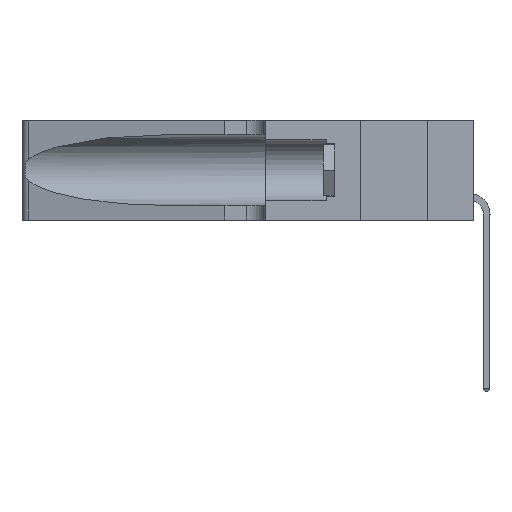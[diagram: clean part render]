
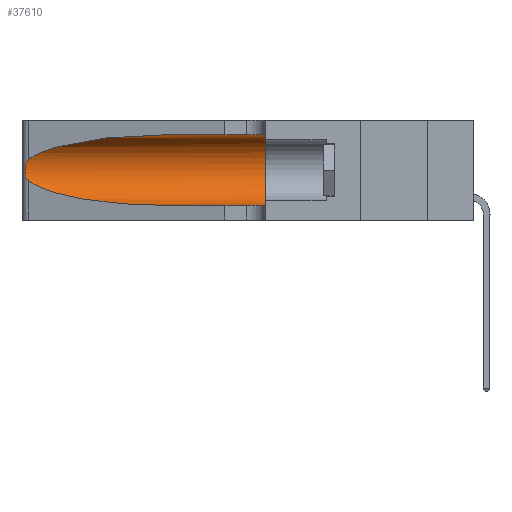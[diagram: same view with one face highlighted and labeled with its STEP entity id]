
A CAD part, left-side view. The second image highlights one B-rep face of the part: STEP entity #37610.
In plain terms, the highlighted cylindrical face has radius 3.308 mm (diameter 6.617 mm), a partial arc.
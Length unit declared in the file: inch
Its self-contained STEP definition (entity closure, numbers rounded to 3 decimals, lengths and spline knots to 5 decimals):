
#437 = CARTESIAN_POINT ( 'NONE',  ( 0.25487, 1.22718, 0.14631 ) ) ;
#970 = VERTEX_POINT ( 'NONE', #36939 ) ;
#1136 = CARTESIAN_POINT ( 'NONE',  ( 0.18966, 0.96281, 0.05475 ) ) ;
#1139 = EDGE_CURVE ( 'NONE', #23087, #42691, #31181, .T. ) ;
#1422 = CARTESIAN_POINT ( 'NONE',  ( 0.2373, 1.15595, 0.08982 ) ) ;
#1552 = ORIENTED_EDGE ( 'NONE', *, *, #41452, .T. ) ;
#1621 = EDGE_CURVE ( 'NONE', #970, #6947, #23301, .T. ) ;
#2358 = CARTESIAN_POINT ( 'NONE',  ( 0.25487, 1.22718, 0.22369 ) ) ;
#2500 = CARTESIAN_POINT ( 'NONE',  ( 0.25639, 1.23186, 0.15144 ) ) ;
#2774 = CARTESIAN_POINT ( 'NONE',  ( 0.1305, 1.61858, 0.05475 ) ) ;
#3064 = DIRECTION ( 'NONE',  ( 0., -1., 0. ) ) ;
#4676 = CARTESIAN_POINT ( 'NONE',  ( 0.1305, 0.72297, 0.05475 ) ) ;
#5617 = EDGE_CURVE ( 'NONE', #6947, #23087, #35823, .T. ) ;
#6044 = VECTOR ( 'NONE', #29354, 39.37008 ) ;
#6947 = VERTEX_POINT ( 'NONE', #34089 ) ;
#9613 = CARTESIAN_POINT ( 'NONE',  ( 0.2373, 1.15595, 0.28018 ) ) ;
#10193 = CARTESIAN_POINT ( 'NONE',  ( 0.1305, 0.72297, 0.31525 ) ) ;
#10388 = ORIENTED_EDGE ( 'NONE', *, *, #5617, .T. ) ;
#11245 = DIRECTION ( 'NONE',  ( 0., 1., 0. ) ) ;
#11796 = AXIS2_PLACEMENT_3D ( 'NONE', #18350, #11245, #21339 ) ;
#12082 = CARTESIAN_POINT ( 'NONE',  ( 0.25555, 1.22994, 0.2215 ) ) ;
#12207 = CARTESIAN_POINT ( 'NONE',  ( 0.1305, 0.35, 0.05475 ) ) ;
#12245 = CARTESIAN_POINT ( 'NONE',  ( 0.1305, 0.35, 0.31525 ) ) ;
#13258 = ORIENTED_EDGE ( 'NONE', *, *, #1621, .T. ) ;
#15030 = LINE ( 'NONE', #15586, #6044 ) ;
#15510 = CARTESIAN_POINT ( 'NONE',  ( 0.26075, 1.23896, 0.178 ) ) ;
#15586 = CARTESIAN_POINT ( 'NONE',  ( 0.1305, 1.61858, 0.31525 ) ) ;
#15776 = DIRECTION ( 'NONE',  ( 0., -1., 0. ) ) ;
#15878 = FACE_OUTER_BOUND ( 'NONE', #30344, .T. ) ;
#18350 = CARTESIAN_POINT ( 'NONE',  ( 0.1305, 0.35, 0.185 ) ) ;
#18883 = CARTESIAN_POINT ( 'NONE',  ( 0.25487, 1.22718, 0.14631 ) ) ;
#19032 = CARTESIAN_POINT ( 'NONE',  ( 0.26017, 1.23833, 0.17102 ) ) ;
#19601 = CARTESIAN_POINT ( 'NONE',  ( 0.1305, 1.61858, 0.185 ) ) ;
#21339 = DIRECTION ( 'NONE',  ( 0., 0., 1. ) ) ;
#22759 = CARTESIAN_POINT ( 'NONE',  ( 0.25854, 1.2359, 0.20912 ) ) ;
#22875 = VERTEX_POINT ( 'NONE', #12245 ) ;
#23087 = VERTEX_POINT ( 'NONE', #437 ) ;
#23244 = CARTESIAN_POINT ( 'NONE',  ( 0.18966, 0.96281, 0.31525 ) ) ;
#23301 =( BOUNDED_CURVE ( )  B_SPLINE_CURVE ( 3, ( #10193, #23244, #9613, #36888 ),
 .UNSPECIFIED., .F., .T. ) 
 B_SPLINE_CURVE_WITH_KNOTS ( ( 4, 4 ),
 ( 1.5708, 2.84003 ),
 .UNSPECIFIED. ) 
 CURVE ( )  GEOMETRIC_REPRESENTATION_ITEM ( )  RATIONAL_B_SPLINE_CURVE ( ( 1., 0.87, 0.87, 1. ) ) 
 REPRESENTATION_ITEM ( '' )  );
#25741 = CARTESIAN_POINT ( 'NONE',  ( 0.25789, 1.23486, 0.15765 ) ) ;
#27096 = ORIENTED_EDGE ( 'NONE', *, *, #28011, .F. ) ;
#27390 = VERTEX_POINT ( 'NONE', #12207 ) ;
#28011 = EDGE_CURVE ( 'NONE', #970, #22875, #15030, .T. ) ;
#28787 = VECTOR ( 'NONE', #3064, 39.37008 ) ;
#29187 = CARTESIAN_POINT ( 'NONE',  ( 0.1305, 0.72297, 0.05475 ) ) ;
#29288 = LINE ( 'NONE', #2774, #28787 ) ;
#29354 = DIRECTION ( 'NONE',  ( 0., -1., 0. ) ) ;
#30344 = EDGE_LOOP ( 'NONE', ( #13258, #10388, #35855, #1552, #39342, #27096 ) ) ;
#31181 =( BOUNDED_CURVE ( )  B_SPLINE_CURVE ( 3, ( #31279, #1422, #1136, #4676 ),
 .UNSPECIFIED., .F., .F. ) 
 B_SPLINE_CURVE_WITH_KNOTS ( ( 4, 4 ),
 ( 3.44316, 4.71239 ),
 .UNSPECIFIED. ) 
 CURVE ( )  GEOMETRIC_REPRESENTATION_ITEM ( )  RATIONAL_B_SPLINE_CURVE ( ( 1., 0.87, 0.87, 1. ) ) 
 REPRESENTATION_ITEM ( '' )  );
#31279 = CARTESIAN_POINT ( 'NONE',  ( 0.25487, 1.22718, 0.14631 ) ) ;
#32405 = CARTESIAN_POINT ( 'NONE',  ( 0.25787, 1.23484, 0.2124 ) ) ;
#32713 = AXIS2_PLACEMENT_3D ( 'NONE', #19601, #15776, #43372 ) ;
#33386 = CYLINDRICAL_SURFACE ( 'NONE', #32713, 0.13025 ) ;
#34089 = CARTESIAN_POINT ( 'NONE',  ( 0.25487, 1.22718, 0.22369 ) ) ;
#35673 = CARTESIAN_POINT ( 'NONE',  ( 0.25639, 1.23184, 0.21858 ) ) ;
#35816 = CARTESIAN_POINT ( 'NONE',  ( 0.26018, 1.23835, 0.19895 ) ) ;
#35823 = B_SPLINE_CURVE_WITH_KNOTS ( 'NONE', 3,
 ( #2358, #12082, #35673, #32405, #22759, #35816, #42516, #15510, #19032, #42665, #25741, #2500, #39250, #18883 ),
 .UNSPECIFIED., .F., .F.,
 ( 4, 2, 2, 2, 2, 2, 4 ),
 ( 0., 0.00027, 0.00053, 0.00107, 0.0016, 0.00187, 0.00214 ),
 .UNSPECIFIED. ) ;
#35855 = ORIENTED_EDGE ( 'NONE', *, *, #1139, .T. ) ;
#36888 = CARTESIAN_POINT ( 'NONE',  ( 0.25487, 1.22718, 0.22369 ) ) ;
#36939 = CARTESIAN_POINT ( 'NONE',  ( 0.1305, 0.72297, 0.31525 ) ) ;
#37610 = ADVANCED_FACE ( 'NONE', ( #15878 ), #33386, .F. ) ;
#39250 = CARTESIAN_POINT ( 'NONE',  ( 0.25555, 1.22993, 0.14849 ) ) ;
#39342 = ORIENTED_EDGE ( 'NONE', *, *, #42448, .F. ) ;
#40337 = CIRCLE ( 'NONE', #11796, 0.13025 ) ;
#41452 = EDGE_CURVE ( 'NONE', #42691, #27390, #29288, .T. ) ;
#42448 = EDGE_CURVE ( 'NONE', #22875, #27390, #40337, .T. ) ;
#42516 = CARTESIAN_POINT ( 'NONE',  ( 0.26075, 1.23896, 0.19203 ) ) ;
#42665 = CARTESIAN_POINT ( 'NONE',  ( 0.25856, 1.23593, 0.16098 ) ) ;
#42691 = VERTEX_POINT ( 'NONE', #29187 ) ;
#43372 = DIRECTION ( 'NONE',  ( 0., 0., -1. ) ) ;
